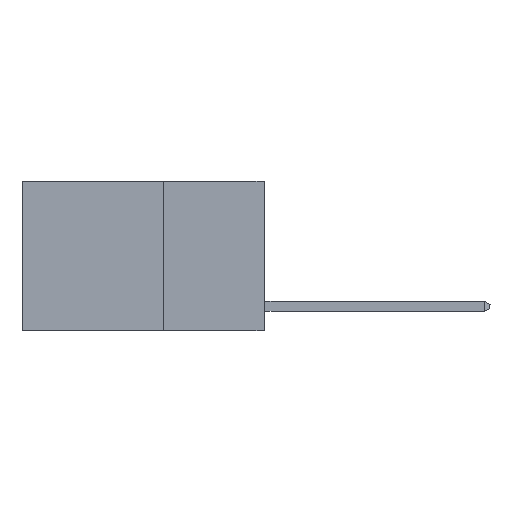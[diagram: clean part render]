
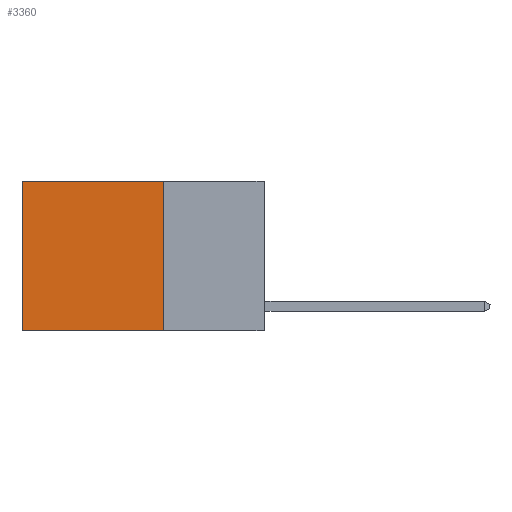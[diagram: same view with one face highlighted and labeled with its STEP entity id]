
A CAD part, left-side view. The second image highlights one B-rep face of the part: STEP entity #3360.
In plain terms, the highlighted planar face has unit normal (-1, 0, 0).
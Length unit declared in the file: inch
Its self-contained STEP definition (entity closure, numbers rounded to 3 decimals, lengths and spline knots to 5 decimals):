
#143 = CARTESIAN_POINT ( 'NONE',  ( 0.2625, 0.25, -0.37 ) ) ;
#302 = EDGE_LOOP ( 'NONE', ( #5059, #6833, #3139, #3867 ) ) ;
#379 = VERTEX_POINT ( 'NONE', #143 ) ;
#522 = CARTESIAN_POINT ( 'NONE',  ( 0.2625, 0.25, 0. ) ) ;
#658 = EDGE_CURVE ( 'NONE', #379, #3031, #6185, .T. ) ;
#838 = VERTEX_POINT ( 'NONE', #10545 ) ;
#1311 = VERTEX_POINT ( 'NONE', #10221 ) ;
#1484 = DIRECTION ( 'NONE',  ( 0., 0., -1. ) ) ;
#1794 = CARTESIAN_POINT ( 'NONE',  ( 0.2625, 0.25, -0.37 ) ) ;
#2033 = VECTOR ( 'NONE', #6635, 39.37008 ) ;
#2539 = VECTOR ( 'NONE', #6662, 39.37008 ) ;
#3031 = VERTEX_POINT ( 'NONE', #5864 ) ;
#3139 = ORIENTED_EDGE ( 'NONE', *, *, #8499, .F. ) ;
#3360 = ADVANCED_FACE ( 'NONE', ( #10097 ), #10238, .F. ) ;
#3737 = AXIS2_PLACEMENT_3D ( 'NONE', #522, #6786, #1484 ) ;
#3867 = ORIENTED_EDGE ( 'NONE', *, *, #6553, .T. ) ;
#3979 = VECTOR ( 'NONE', #6681, 39.37008 ) ;
#5010 = LINE ( 'NONE', #10140, #2539 ) ;
#5059 = ORIENTED_EDGE ( 'NONE', *, *, #9384, .T. ) ;
#5864 = CARTESIAN_POINT ( 'NONE',  ( 0.2625, 0.6, -0.37 ) ) ;
#5953 = DIRECTION ( 'NONE',  ( 0., 0., -1. ) ) ;
#6185 = LINE ( 'NONE', #1794, #3979 ) ;
#6356 = VECTOR ( 'NONE', #5953, 39.37008 ) ;
#6553 = EDGE_CURVE ( 'NONE', #838, #1311, #5010, .T. ) ;
#6635 = DIRECTION ( 'NONE',  ( 0., 0., -1. ) ) ;
#6662 = DIRECTION ( 'NONE',  ( 0., 1., 0. ) ) ;
#6681 = DIRECTION ( 'NONE',  ( 0., 1., 0. ) ) ;
#6786 = DIRECTION ( 'NONE',  ( 1., 0., 0. ) ) ;
#6833 = ORIENTED_EDGE ( 'NONE', *, *, #658, .F. ) ;
#8125 = CARTESIAN_POINT ( 'NONE',  ( 0.2625, 0.25, 0. ) ) ;
#8275 = LINE ( 'NONE', #8125, #6356 ) ;
#8374 = LINE ( 'NONE', #10116, #2033 ) ;
#8499 = EDGE_CURVE ( 'NONE', #838, #379, #8275, .T. ) ;
#9384 = EDGE_CURVE ( 'NONE', #1311, #3031, #8374, .T. ) ;
#10097 = FACE_OUTER_BOUND ( 'NONE', #302, .T. ) ;
#10116 = CARTESIAN_POINT ( 'NONE',  ( 0.2625, 0.6, 0. ) ) ;
#10140 = CARTESIAN_POINT ( 'NONE',  ( 0.2625, 0.25, 0. ) ) ;
#10221 = CARTESIAN_POINT ( 'NONE',  ( 0.2625, 0.6, 0. ) ) ;
#10238 = PLANE ( 'NONE',  #3737 ) ;
#10545 = CARTESIAN_POINT ( 'NONE',  ( 0.2625, 0.25, 0. ) ) ;
